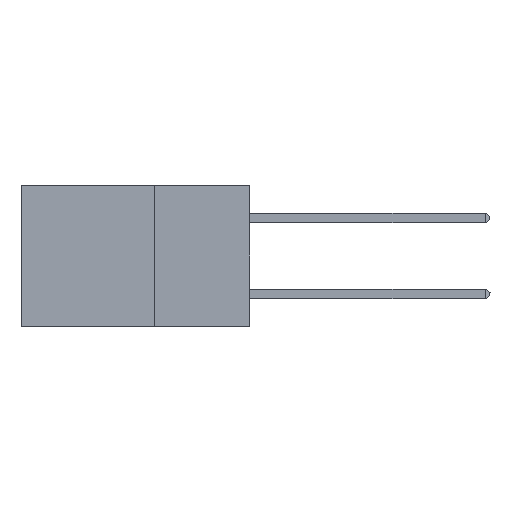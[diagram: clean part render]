
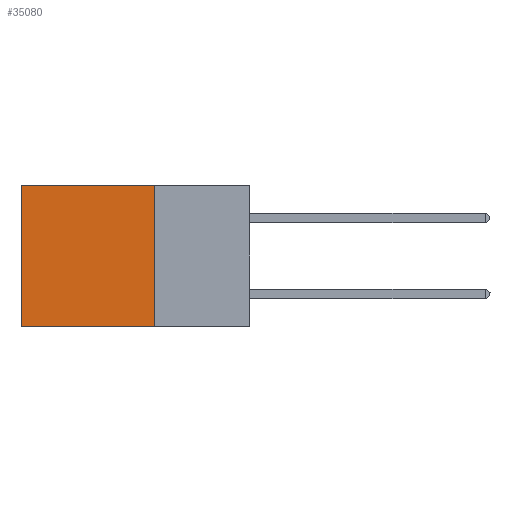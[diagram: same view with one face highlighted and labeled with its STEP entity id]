
A CAD part, left-side view. The second image highlights one B-rep face of the part: STEP entity #35080.
In plain terms, the highlighted planar face has unit normal (-1, 0, 0).
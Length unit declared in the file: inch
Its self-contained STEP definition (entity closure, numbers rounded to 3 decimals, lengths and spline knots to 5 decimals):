
#153 = LINE ( 'NONE', #6846, #21308 ) ;
#516 = DIRECTION ( 'NONE',  ( 0., 0., -1. ) ) ;
#6265 = CARTESIAN_POINT ( 'NONE',  ( 0.2875, 0.25, 0. ) ) ;
#6846 = CARTESIAN_POINT ( 'NONE',  ( 0.2875, 0.25, 0. ) ) ;
#8427 = VECTOR ( 'NONE', #12584, 39.37008 ) ;
#9067 = ORIENTED_EDGE ( 'NONE', *, *, #19720, .F. ) ;
#10315 = DIRECTION ( 'NONE',  ( 1., 0., 0. ) ) ;
#12145 = EDGE_LOOP ( 'NONE', ( #28816, #14817, #9067, #27479 ) ) ;
#12584 = DIRECTION ( 'NONE',  ( 0., 1., 0. ) ) ;
#12998 = VERTEX_POINT ( 'NONE', #39891 ) ;
#13059 = DIRECTION ( 'NONE',  ( 0., 1., 0. ) ) ;
#13485 = CARTESIAN_POINT ( 'NONE',  ( 0.2875, 0.25, 0. ) ) ;
#14701 = VERTEX_POINT ( 'NONE', #16432 ) ;
#14817 = ORIENTED_EDGE ( 'NONE', *, *, #37512, .F. ) ;
#14820 = LINE ( 'NONE', #6265, #31372 ) ;
#16432 = CARTESIAN_POINT ( 'NONE',  ( 0.2875, 0.25, -0.37 ) ) ;
#17716 = DIRECTION ( 'NONE',  ( 0., 0., -1. ) ) ;
#18680 = VECTOR ( 'NONE', #17716, 39.37008 ) ;
#19720 = EDGE_CURVE ( 'NONE', #31581, #14701, #153, .T. ) ;
#20131 = DIRECTION ( 'NONE',  ( 0., 0., -1. ) ) ;
#20782 = CARTESIAN_POINT ( 'NONE',  ( 0.2875, 0.25, 0. ) ) ;
#21308 = VECTOR ( 'NONE', #516, 39.37008 ) ;
#22521 = EDGE_CURVE ( 'NONE', #12998, #28954, #27452, .T. ) ;
#24922 = CARTESIAN_POINT ( 'NONE',  ( 0.2875, 0.6, 0. ) ) ;
#27452 = LINE ( 'NONE', #24922, #18680 ) ;
#27479 = ORIENTED_EDGE ( 'NONE', *, *, #39908, .T. ) ;
#28816 = ORIENTED_EDGE ( 'NONE', *, *, #22521, .T. ) ;
#28954 = VERTEX_POINT ( 'NONE', #33589 ) ;
#31330 = FACE_OUTER_BOUND ( 'NONE', #12145, .T. ) ;
#31372 = VECTOR ( 'NONE', #13059, 39.37008 ) ;
#31581 = VERTEX_POINT ( 'NONE', #20782 ) ;
#32714 = CARTESIAN_POINT ( 'NONE',  ( 0.2875, 0.25, -0.37 ) ) ;
#33466 = PLANE ( 'NONE',  #34085 ) ;
#33589 = CARTESIAN_POINT ( 'NONE',  ( 0.2875, 0.6, -0.37 ) ) ;
#34085 = AXIS2_PLACEMENT_3D ( 'NONE', #13485, #10315, #20131 ) ;
#35080 = ADVANCED_FACE ( 'NONE', ( #31330 ), #33466, .F. ) ;
#37512 = EDGE_CURVE ( 'NONE', #14701, #28954, #39465, .T. ) ;
#39465 = LINE ( 'NONE', #32714, #8427 ) ;
#39891 = CARTESIAN_POINT ( 'NONE',  ( 0.2875, 0.6, 0. ) ) ;
#39908 = EDGE_CURVE ( 'NONE', #31581, #12998, #14820, .T. ) ;
